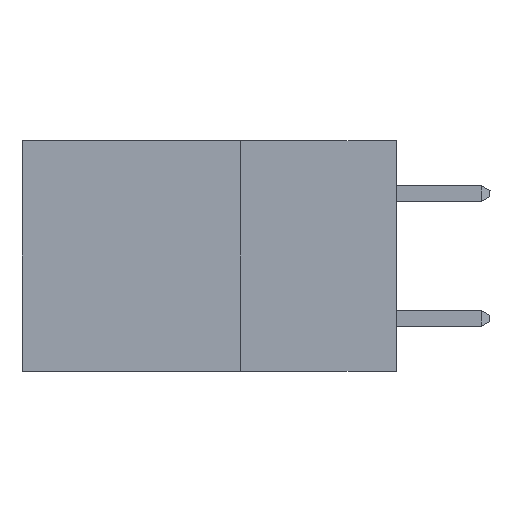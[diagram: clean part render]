
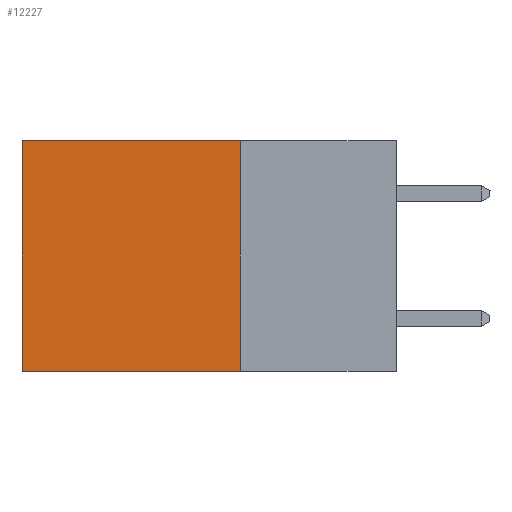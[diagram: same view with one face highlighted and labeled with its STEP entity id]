
A CAD part, left-side view. The second image highlights one B-rep face of the part: STEP entity #12227.
In plain terms, the highlighted planar face has unit normal (-1, 0, 0).
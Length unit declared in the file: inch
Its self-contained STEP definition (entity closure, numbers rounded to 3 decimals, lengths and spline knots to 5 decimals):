
#295 = CARTESIAN_POINT ( 'NONE',  ( 0.298, 0.6, 0. ) ) ;
#1188 = LINE ( 'NONE', #17281, #13021 ) ;
#1253 = CARTESIAN_POINT ( 'NONE',  ( 0.298, 0.6, 0. ) ) ;
#2490 = CARTESIAN_POINT ( 'NONE',  ( 0.298, 0.6, -0.37 ) ) ;
#2580 = PLANE ( 'NONE',  #6811 ) ;
#3094 = DIRECTION ( 'NONE',  ( 0., 1., 0. ) ) ;
#3303 = DIRECTION ( 'NONE',  ( 0., 0., -1. ) ) ;
#3994 = LINE ( 'NONE', #7508, #15680 ) ;
#4020 = CARTESIAN_POINT ( 'NONE',  ( 0.298, 0.25, 0. ) ) ;
#5512 = DIRECTION ( 'NONE',  ( 1., 0., 0. ) ) ;
#5712 = VERTEX_POINT ( 'NONE', #1253 ) ;
#6060 = VECTOR ( 'NONE', #3303, 39.37008 ) ;
#6294 = EDGE_LOOP ( 'NONE', ( #6862, #7081, #7614, #7671 ) ) ;
#6811 = AXIS2_PLACEMENT_3D ( 'NONE', #4020, #5512, #15279 ) ;
#6862 = ORIENTED_EDGE ( 'NONE', *, *, #9215, .T. ) ;
#7016 = CARTESIAN_POINT ( 'NONE',  ( 0.298, 0.25, -0.37 ) ) ;
#7081 = ORIENTED_EDGE ( 'NONE', *, *, #11750, .F. ) ;
#7309 = LINE ( 'NONE', #8837, #14711 ) ;
#7508 = CARTESIAN_POINT ( 'NONE',  ( 0.298, 0.25, 0. ) ) ;
#7578 = DIRECTION ( 'NONE',  ( 0., 1., 0. ) ) ;
#7614 = ORIENTED_EDGE ( 'NONE', *, *, #9121, .F. ) ;
#7662 = VERTEX_POINT ( 'NONE', #7016 ) ;
#7671 = ORIENTED_EDGE ( 'NONE', *, *, #11038, .T. ) ;
#8837 = CARTESIAN_POINT ( 'NONE',  ( 0.298, 0.25, -0.37 ) ) ;
#9121 = EDGE_CURVE ( 'NONE', #9340, #7662, #3994, .T. ) ;
#9215 = EDGE_CURVE ( 'NONE', #5712, #15933, #9840, .T. ) ;
#9340 = VERTEX_POINT ( 'NONE', #16252 ) ;
#9840 = LINE ( 'NONE', #295, #6060 ) ;
#11038 = EDGE_CURVE ( 'NONE', #9340, #5712, #1188, .T. ) ;
#11750 = EDGE_CURVE ( 'NONE', #7662, #15933, #7309, .T. ) ;
#12227 = ADVANCED_FACE ( 'NONE', ( #13840 ), #2580, .F. ) ;
#13021 = VECTOR ( 'NONE', #7578, 39.37008 ) ;
#13840 = FACE_OUTER_BOUND ( 'NONE', #6294, .T. ) ;
#14711 = VECTOR ( 'NONE', #3094, 39.37008 ) ;
#15279 = DIRECTION ( 'NONE',  ( 0., 0., -1. ) ) ;
#15680 = VECTOR ( 'NONE', #17220, 39.37008 ) ;
#15933 = VERTEX_POINT ( 'NONE', #2490 ) ;
#16252 = CARTESIAN_POINT ( 'NONE',  ( 0.298, 0.25, 0. ) ) ;
#17220 = DIRECTION ( 'NONE',  ( 0., 0., -1. ) ) ;
#17281 = CARTESIAN_POINT ( 'NONE',  ( 0.298, 0.25, 0. ) ) ;
